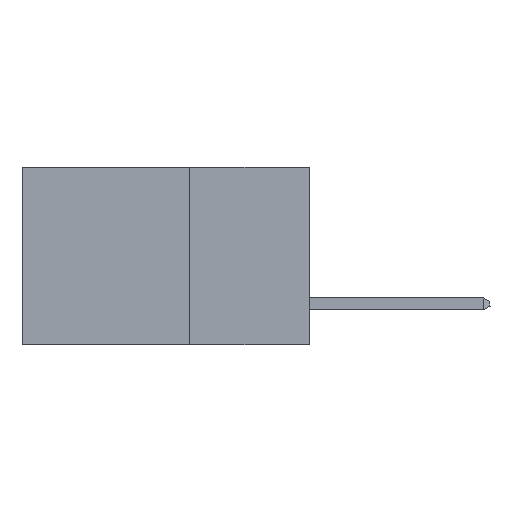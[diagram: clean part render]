
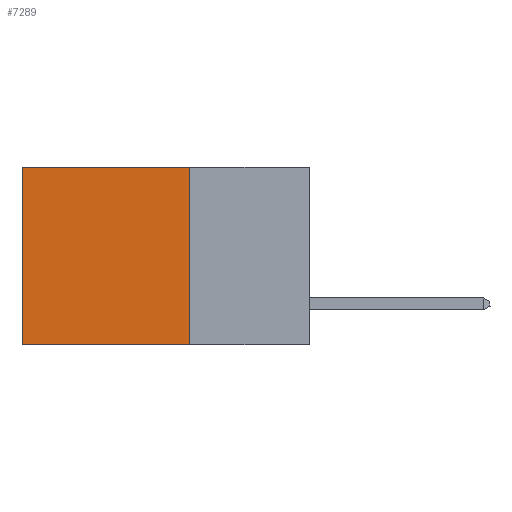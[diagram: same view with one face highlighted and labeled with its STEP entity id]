
A CAD part, left-side view. The second image highlights one B-rep face of the part: STEP entity #7289.
In plain terms, the highlighted planar face has unit normal (-1, 0, 0).
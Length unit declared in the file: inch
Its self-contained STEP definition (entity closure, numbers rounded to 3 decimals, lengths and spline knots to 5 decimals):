
#331 = CARTESIAN_POINT ( 'NONE',  ( 0.2875, 0.25, 0. ) ) ;
#826 = CARTESIAN_POINT ( 'NONE',  ( 0.2875, 0.25, -0.37 ) ) ;
#1182 = DIRECTION ( 'NONE',  ( 0., 1., 0. ) ) ;
#1220 = PLANE ( 'NONE',  #3995 ) ;
#1299 = CARTESIAN_POINT ( 'NONE',  ( 0.2875, 0.25, -0.37 ) ) ;
#1474 = DIRECTION ( 'NONE',  ( 1., 0., 0. ) ) ;
#1775 = VERTEX_POINT ( 'NONE', #1299 ) ;
#2045 = CARTESIAN_POINT ( 'NONE',  ( 0.2875, 0.25, 0. ) ) ;
#2292 = VECTOR ( 'NONE', #2406, 39.37008 ) ;
#2406 = DIRECTION ( 'NONE',  ( 0., 1., 0. ) ) ;
#2503 = FACE_OUTER_BOUND ( 'NONE', #5221, .T. ) ;
#2534 = EDGE_CURVE ( 'NONE', #9574, #5325, #7518, .T. ) ;
#2656 = ORIENTED_EDGE ( 'NONE', *, *, #3134, .F. ) ;
#3134 = EDGE_CURVE ( 'NONE', #6017, #1775, #10195, .T. ) ;
#3606 = LINE ( 'NONE', #826, #2292 ) ;
#3766 = CARTESIAN_POINT ( 'NONE',  ( 0.2875, 0.25, 0. ) ) ;
#3972 = CARTESIAN_POINT ( 'NONE',  ( 0.2875, 0.6, 0. ) ) ;
#3995 = AXIS2_PLACEMENT_3D ( 'NONE', #2045, #1474, #7088 ) ;
#4030 = ORIENTED_EDGE ( 'NONE', *, *, #7165, .T. ) ;
#5131 = ORIENTED_EDGE ( 'NONE', *, *, #9773, .F. ) ;
#5221 = EDGE_LOOP ( 'NONE', ( #9935, #5131, #2656, #4030 ) ) ;
#5325 = VERTEX_POINT ( 'NONE', #10023 ) ;
#5853 = VECTOR ( 'NONE', #10373, 39.37008 ) ;
#5867 = LINE ( 'NONE', #331, #9448 ) ;
#6017 = VERTEX_POINT ( 'NONE', #9154 ) ;
#7009 = DIRECTION ( 'NONE',  ( 0., 0., -1. ) ) ;
#7088 = DIRECTION ( 'NONE',  ( 0., 0., -1. ) ) ;
#7165 = EDGE_CURVE ( 'NONE', #6017, #9574, #5867, .T. ) ;
#7289 = ADVANCED_FACE ( 'NONE', ( #2503 ), #1220, .F. ) ;
#7518 = LINE ( 'NONE', #9481, #10079 ) ;
#9154 = CARTESIAN_POINT ( 'NONE',  ( 0.2875, 0.25, 0. ) ) ;
#9448 = VECTOR ( 'NONE', #1182, 39.37008 ) ;
#9481 = CARTESIAN_POINT ( 'NONE',  ( 0.2875, 0.6, 0. ) ) ;
#9574 = VERTEX_POINT ( 'NONE', #3972 ) ;
#9773 = EDGE_CURVE ( 'NONE', #1775, #5325, #3606, .T. ) ;
#9935 = ORIENTED_EDGE ( 'NONE', *, *, #2534, .T. ) ;
#10023 = CARTESIAN_POINT ( 'NONE',  ( 0.2875, 0.6, -0.37 ) ) ;
#10079 = VECTOR ( 'NONE', #7009, 39.37008 ) ;
#10195 = LINE ( 'NONE', #3766, #5853 ) ;
#10373 = DIRECTION ( 'NONE',  ( 0., 0., -1. ) ) ;
